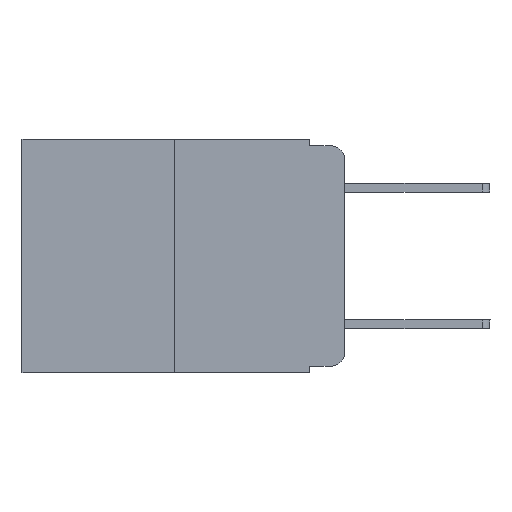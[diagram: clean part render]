
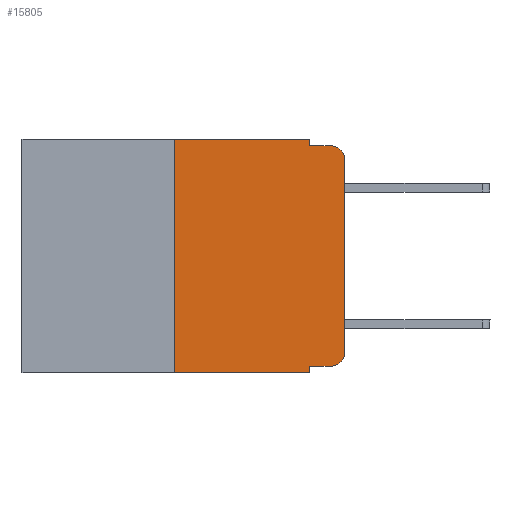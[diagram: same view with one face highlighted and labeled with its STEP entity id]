
A CAD part, left-side view. The second image highlights one B-rep face of the part: STEP entity #15805.
In plain terms, the highlighted planar face has unit normal (-1, 0, 0).
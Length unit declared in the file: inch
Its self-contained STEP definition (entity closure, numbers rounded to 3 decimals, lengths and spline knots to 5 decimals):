
#60 = CARTESIAN_POINT ( 'NONE',  ( 0., 0.25, 0. ) ) ;
#292 = EDGE_CURVE ( 'NONE', #6855, #4398, #12413, .T. ) ;
#528 = VERTEX_POINT ( 'NONE', #3368 ) ;
#700 = VERTEX_POINT ( 'NONE', #8757 ) ;
#803 = LINE ( 'NONE', #3952, #12096 ) ;
#980 = EDGE_CURVE ( 'NONE', #18126, #6569, #11638, .T. ) ;
#1012 = ORIENTED_EDGE ( 'NONE', *, *, #5156, .T. ) ;
#1717 = EDGE_CURVE ( 'NONE', #4398, #6569, #15088, .T. ) ;
#2117 = CARTESIAN_POINT ( 'NONE',  ( 0., 0.25, 0. ) ) ;
#3032 = AXIS2_PLACEMENT_3D ( 'NONE', #7430, #18509, #7850 ) ;
#3368 = CARTESIAN_POINT ( 'NONE',  ( 0., 0.02, -0.333 ) ) ;
#3490 = VERTEX_POINT ( 'NONE', #7187 ) ;
#3690 = DIRECTION ( 'NONE',  ( 0., 0., 1. ) ) ;
#3899 = VECTOR ( 'NONE', #7306, 39.37008 ) ;
#3947 = DIRECTION ( 'NONE',  ( 0., -1., 0. ) ) ;
#3952 = CARTESIAN_POINT ( 'NONE',  ( 0., 0.051, -0.333 ) ) ;
#4144 = ORIENTED_EDGE ( 'NONE', *, *, #9779, .F. ) ;
#4281 = CARTESIAN_POINT ( 'NONE',  ( 0., 0.051, 0. ) ) ;
#4398 = VERTEX_POINT ( 'NONE', #6515 ) ;
#5156 = EDGE_CURVE ( 'NONE', #700, #528, #803, .T. ) ;
#5767 = DIRECTION ( 'NONE',  ( 0., 0., -1. ) ) ;
#5839 = DIRECTION ( 'NONE',  ( 0., 0., -1. ) ) ;
#6420 = LINE ( 'NONE', #2117, #9406 ) ;
#6444 = VECTOR ( 'NONE', #20220, 39.37008 ) ;
#6515 = CARTESIAN_POINT ( 'NONE',  ( 0., 0.051, -0.01 ) ) ;
#6569 = VERTEX_POINT ( 'NONE', #17242 ) ;
#6855 = VERTEX_POINT ( 'NONE', #4281 ) ;
#6889 = VECTOR ( 'NONE', #3947, 39.37008 ) ;
#7109 = ORIENTED_EDGE ( 'NONE', *, *, #7110, .F. ) ;
#7110 = EDGE_CURVE ( 'NONE', #17188, #6855, #8357, .T. ) ;
#7187 = CARTESIAN_POINT ( 'NONE',  ( 0., 0.25, -0.343 ) ) ;
#7247 = VECTOR ( 'NONE', #5839, 39.37008 ) ;
#7306 = DIRECTION ( 'NONE',  ( 0., -1., 0. ) ) ;
#7430 = CARTESIAN_POINT ( 'NONE',  ( 0., 0.02, -0.03 ) ) ;
#7850 = DIRECTION ( 'NONE',  ( 0., 0., -1. ) ) ;
#8118 = VERTEX_POINT ( 'NONE', #10423 ) ;
#8228 = DIRECTION ( 'NONE',  ( 0., 0., -1. ) ) ;
#8357 = LINE ( 'NONE', #13468, #3899 ) ;
#8425 = ORIENTED_EDGE ( 'NONE', *, *, #292, .F. ) ;
#8757 = CARTESIAN_POINT ( 'NONE',  ( 0., 0.051, -0.333 ) ) ;
#9071 = CARTESIAN_POINT ( 'NONE',  ( 0., 0.473, 0. ) ) ;
#9406 = VECTOR ( 'NONE', #3690, 39.37008 ) ;
#9514 = LINE ( 'NONE', #17455, #18977 ) ;
#9725 = DIRECTION ( 'NONE',  ( 0., 0., 1. ) ) ;
#9775 = ORIENTED_EDGE ( 'NONE', *, *, #1717, .F. ) ;
#9779 = EDGE_CURVE ( 'NONE', #3490, #17188, #6420, .T. ) ;
#10423 = CARTESIAN_POINT ( 'NONE',  ( 0., 0., -0.313 ) ) ;
#10580 = ORIENTED_EDGE ( 'NONE', *, *, #980, .T. ) ;
#10615 = EDGE_CURVE ( 'NONE', #3490, #14216, #20280, .T. ) ;
#10955 = ORIENTED_EDGE ( 'NONE', *, *, #19443, .F. ) ;
#11583 = ORIENTED_EDGE ( 'NONE', *, *, #10615, .T. ) ;
#11638 = CIRCLE ( 'NONE', #3032, 0.02 ) ;
#11851 = DIRECTION ( 'NONE',  ( 0., -1., 0. ) ) ;
#12096 = VECTOR ( 'NONE', #11851, 39.37008 ) ;
#12157 = ORIENTED_EDGE ( 'NONE', *, *, #16412, .T. ) ;
#12164 = DIRECTION ( 'NONE',  ( -1., 0., 0. ) ) ;
#12188 = DIRECTION ( 'NONE',  ( 0., 0., -1. ) ) ;
#12413 = LINE ( 'NONE', #20133, #7247 ) ;
#13354 = CARTESIAN_POINT ( 'NONE',  ( 0., 0.473, -0.343 ) ) ;
#13468 = CARTESIAN_POINT ( 'NONE',  ( 0., 0.473, 0. ) ) ;
#14216 = VERTEX_POINT ( 'NONE', #19457 ) ;
#14297 = AXIS2_PLACEMENT_3D ( 'NONE', #20128, #12164, #5767 ) ;
#14672 = CARTESIAN_POINT ( 'NONE',  ( 0., 0., -0.03 ) ) ;
#14716 = ORIENTED_EDGE ( 'NONE', *, *, #19383, .T. ) ;
#14935 = LINE ( 'NONE', #16034, #15190 ) ;
#15088 = LINE ( 'NONE', #16461, #6444 ) ;
#15190 = VECTOR ( 'NONE', #8228, 39.37008 ) ;
#15805 = ADVANCED_FACE ( 'NONE', ( #18373 ), #18417, .F. ) ;
#16034 = CARTESIAN_POINT ( 'NONE',  ( 0., 0.051, 0. ) ) ;
#16083 = CIRCLE ( 'NONE', #14297, 0.02 ) ;
#16412 = EDGE_CURVE ( 'NONE', #528, #8118, #16083, .T. ) ;
#16461 = CARTESIAN_POINT ( 'NONE',  ( 0., 0.051, -0.01 ) ) ;
#17188 = VERTEX_POINT ( 'NONE', #60 ) ;
#17189 = DIRECTION ( 'NONE',  ( 1., 0., 0. ) ) ;
#17242 = CARTESIAN_POINT ( 'NONE',  ( 0., 0.02, -0.01 ) ) ;
#17455 = CARTESIAN_POINT ( 'NONE',  ( 0., 0., 0. ) ) ;
#18126 = VERTEX_POINT ( 'NONE', #14672 ) ;
#18190 = EDGE_LOOP ( 'NONE', ( #14716, #10580, #9775, #8425, #7109, #4144, #11583, #10955, #1012, #12157 ) ) ;
#18373 = FACE_OUTER_BOUND ( 'NONE', #18190, .T. ) ;
#18417 = PLANE ( 'NONE',  #19115 ) ;
#18509 = DIRECTION ( 'NONE',  ( -1., 0., 0. ) ) ;
#18977 = VECTOR ( 'NONE', #9725, 39.37008 ) ;
#19115 = AXIS2_PLACEMENT_3D ( 'NONE', #9071, #17189, #12188 ) ;
#19383 = EDGE_CURVE ( 'NONE', #8118, #18126, #9514, .T. ) ;
#19443 = EDGE_CURVE ( 'NONE', #700, #14216, #14935, .T. ) ;
#19457 = CARTESIAN_POINT ( 'NONE',  ( 0., 0.051, -0.343 ) ) ;
#20128 = CARTESIAN_POINT ( 'NONE',  ( 0., 0.02, -0.313 ) ) ;
#20133 = CARTESIAN_POINT ( 'NONE',  ( 0., 0.051, 0. ) ) ;
#20220 = DIRECTION ( 'NONE',  ( 0., -1., 0. ) ) ;
#20280 = LINE ( 'NONE', #13354, #6889 ) ;
